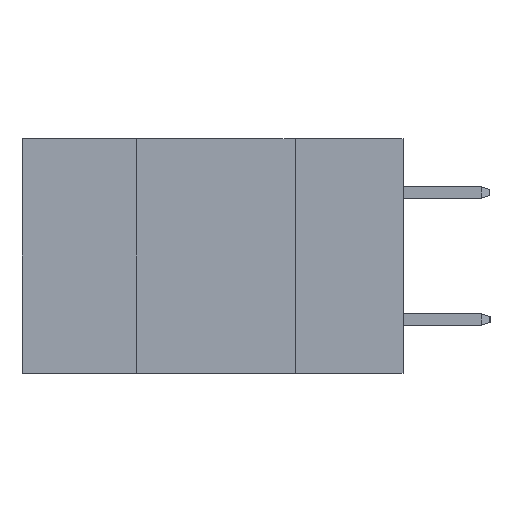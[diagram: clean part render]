
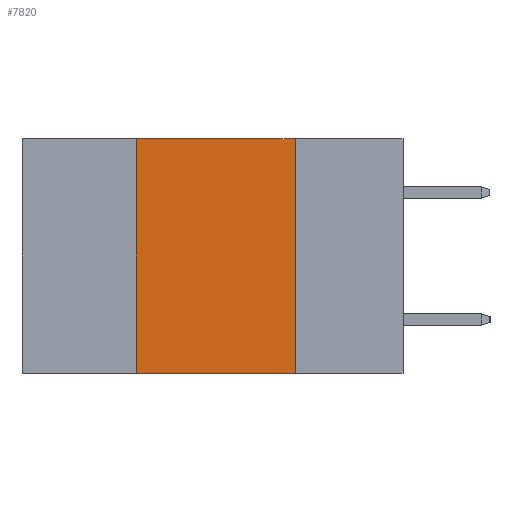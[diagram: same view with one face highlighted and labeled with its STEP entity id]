
A CAD part, left-side view. The second image highlights one B-rep face of the part: STEP entity #7820.
In plain terms, the highlighted planar face has unit normal (-1, 0, 0).
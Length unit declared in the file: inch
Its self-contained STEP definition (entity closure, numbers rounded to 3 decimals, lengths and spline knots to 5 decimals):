
#77 = CARTESIAN_POINT ( 'NONE',  ( 0., 0.6, 0. ) ) ;
#723 = VERTEX_POINT ( 'NONE', #9326 ) ;
#1391 = CARTESIAN_POINT ( 'NONE',  ( 0., 0.42, 0. ) ) ;
#1469 = EDGE_LOOP ( 'NONE', ( #5515, #11807, #17702, #13337 ) ) ;
#2500 = DIRECTION ( 'NONE',  ( 1., 0., 0. ) ) ;
#2702 = EDGE_CURVE ( 'NONE', #9206, #15184, #5103, .T. ) ;
#3001 = LINE ( 'NONE', #77, #20018 ) ;
#4236 = DIRECTION ( 'NONE',  ( 0., 0., -1. ) ) ;
#5103 = LINE ( 'NONE', #14641, #9229 ) ;
#5227 = LINE ( 'NONE', #8976, #6053 ) ;
#5515 = ORIENTED_EDGE ( 'NONE', *, *, #13355, .F. ) ;
#6053 = VECTOR ( 'NONE', #18515, 39.37008 ) ;
#7820 = ADVANCED_FACE ( 'NONE', ( #12449 ), #17279, .F. ) ;
#8202 = CARTESIAN_POINT ( 'NONE',  ( 0., 0.17, -0.37 ) ) ;
#8902 = DIRECTION ( 'NONE',  ( 0., 0., -1. ) ) ;
#8976 = CARTESIAN_POINT ( 'NONE',  ( 0., 0.42, 0. ) ) ;
#9206 = VERTEX_POINT ( 'NONE', #12549 ) ;
#9229 = VECTOR ( 'NONE', #11614, 39.37008 ) ;
#9326 = CARTESIAN_POINT ( 'NONE',  ( 0., 0.17, 0. ) ) ;
#11047 = EDGE_CURVE ( 'NONE', #13844, #723, #3001, .T. ) ;
#11614 = DIRECTION ( 'NONE',  ( 0., -1., 0. ) ) ;
#11807 = ORIENTED_EDGE ( 'NONE', *, *, #11047, .F. ) ;
#12449 = FACE_OUTER_BOUND ( 'NONE', #1469, .T. ) ;
#12549 = CARTESIAN_POINT ( 'NONE',  ( 0., 0.42, -0.37 ) ) ;
#13337 = ORIENTED_EDGE ( 'NONE', *, *, #2702, .T. ) ;
#13355 = EDGE_CURVE ( 'NONE', #723, #15184, #16824, .T. ) ;
#13844 = VERTEX_POINT ( 'NONE', #1391 ) ;
#14641 = CARTESIAN_POINT ( 'NONE',  ( 0., 0.6, -0.37 ) ) ;
#15184 = VERTEX_POINT ( 'NONE', #8202 ) ;
#16228 = AXIS2_PLACEMENT_3D ( 'NONE', #20024, #2500, #8902 ) ;
#16824 = LINE ( 'NONE', #17029, #18548 ) ;
#17029 = CARTESIAN_POINT ( 'NONE',  ( 0., 0.17, 0. ) ) ;
#17138 = EDGE_CURVE ( 'NONE', #9206, #13844, #5227, .T. ) ;
#17279 = PLANE ( 'NONE',  #16228 ) ;
#17702 = ORIENTED_EDGE ( 'NONE', *, *, #17138, .F. ) ;
#17786 = DIRECTION ( 'NONE',  ( 0., -1., 0. ) ) ;
#18515 = DIRECTION ( 'NONE',  ( 0., 0., 1. ) ) ;
#18548 = VECTOR ( 'NONE', #4236, 39.37008 ) ;
#20018 = VECTOR ( 'NONE', #17786, 39.37008 ) ;
#20024 = CARTESIAN_POINT ( 'NONE',  ( 0., 0.6, 0. ) ) ;
